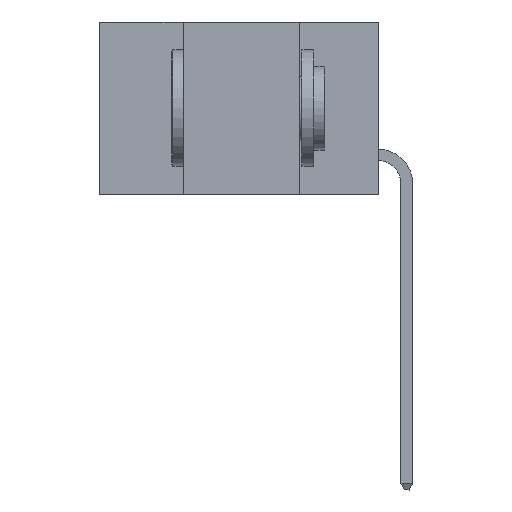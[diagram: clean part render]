
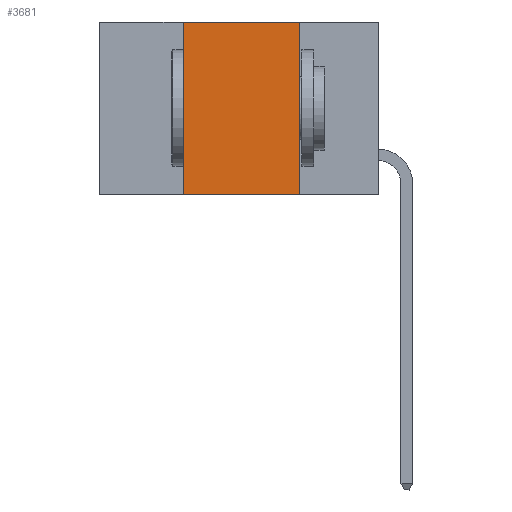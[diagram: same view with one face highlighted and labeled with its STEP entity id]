
A CAD part, left-side view. The second image highlights one B-rep face of the part: STEP entity #3681.
In plain terms, the highlighted planar face has unit normal (-1, 0, 0).
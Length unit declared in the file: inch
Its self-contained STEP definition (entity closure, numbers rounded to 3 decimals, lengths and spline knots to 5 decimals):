
#48 = CARTESIAN_POINT ( 'NONE',  ( 0., 0.17, 0. ) ) ;
#157 = DIRECTION ( 'NONE',  ( 1., 0., 0. ) ) ;
#189 = EDGE_CURVE ( 'NONE', #6704, #3718, #3177, .T. ) ;
#651 = ORIENTED_EDGE ( 'NONE', *, *, #5230, .F. ) ;
#1053 = VERTEX_POINT ( 'NONE', #4760 ) ;
#1265 = LINE ( 'NONE', #1370, #5181 ) ;
#1370 = CARTESIAN_POINT ( 'NONE',  ( 0., 0.6, -0.37 ) ) ;
#2426 = CARTESIAN_POINT ( 'NONE',  ( 0., 0.6, 0. ) ) ;
#2431 = LINE ( 'NONE', #6803, #8635 ) ;
#2570 = EDGE_LOOP ( 'NONE', ( #7475, #2661, #651, #3295 ) ) ;
#2614 = DIRECTION ( 'NONE',  ( 0., 0., -1. ) ) ;
#2661 = ORIENTED_EDGE ( 'NONE', *, *, #189, .F. ) ;
#3119 = VECTOR ( 'NONE', #4154, 39.37008 ) ;
#3177 = LINE ( 'NONE', #2426, #3119 ) ;
#3295 = ORIENTED_EDGE ( 'NONE', *, *, #5507, .T. ) ;
#3681 = ADVANCED_FACE ( 'NONE', ( #7110 ), #9605, .F. ) ;
#3718 = VERTEX_POINT ( 'NONE', #48 ) ;
#4154 = DIRECTION ( 'NONE',  ( 0., -1., 0. ) ) ;
#4507 = DIRECTION ( 'NONE',  ( 0., 0., -1. ) ) ;
#4673 = DIRECTION ( 'NONE',  ( 0., -1., 0. ) ) ;
#4760 = CARTESIAN_POINT ( 'NONE',  ( 0., 0.42, -0.37 ) ) ;
#5181 = VECTOR ( 'NONE', #4673, 39.37008 ) ;
#5230 = EDGE_CURVE ( 'NONE', #1053, #6704, #2431, .T. ) ;
#5507 = EDGE_CURVE ( 'NONE', #1053, #7424, #1265, .T. ) ;
#5908 = DIRECTION ( 'NONE',  ( 0., 0., 1. ) ) ;
#6078 = CARTESIAN_POINT ( 'NONE',  ( 0., 0.6, 0. ) ) ;
#6704 = VERTEX_POINT ( 'NONE', #8126 ) ;
#6803 = CARTESIAN_POINT ( 'NONE',  ( 0., 0.42, -0.37 ) ) ;
#7110 = FACE_OUTER_BOUND ( 'NONE', #2570, .T. ) ;
#7424 = VERTEX_POINT ( 'NONE', #8097 ) ;
#7475 = ORIENTED_EDGE ( 'NONE', *, *, #9952, .F. ) ;
#7795 = CARTESIAN_POINT ( 'NONE',  ( 0., 0.17, -0.37 ) ) ;
#8097 = CARTESIAN_POINT ( 'NONE',  ( 0., 0.17, -0.37 ) ) ;
#8126 = CARTESIAN_POINT ( 'NONE',  ( 0., 0.42, 0. ) ) ;
#8600 = LINE ( 'NONE', #7795, #9951 ) ;
#8635 = VECTOR ( 'NONE', #5908, 39.37008 ) ;
#9605 = PLANE ( 'NONE',  #10049 ) ;
#9951 = VECTOR ( 'NONE', #2614, 39.37008 ) ;
#9952 = EDGE_CURVE ( 'NONE', #3718, #7424, #8600, .T. ) ;
#10049 = AXIS2_PLACEMENT_3D ( 'NONE', #6078, #157, #4507 ) ;
